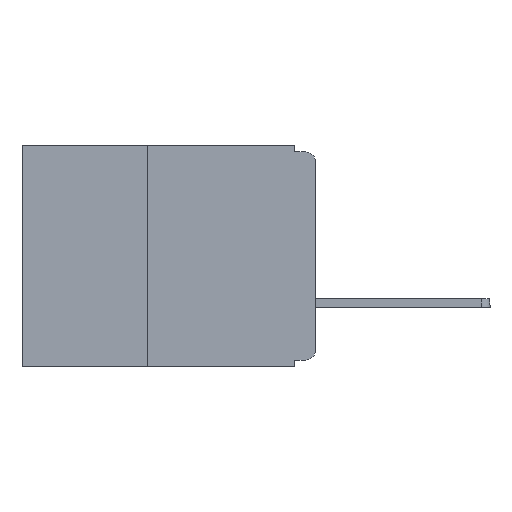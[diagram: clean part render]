
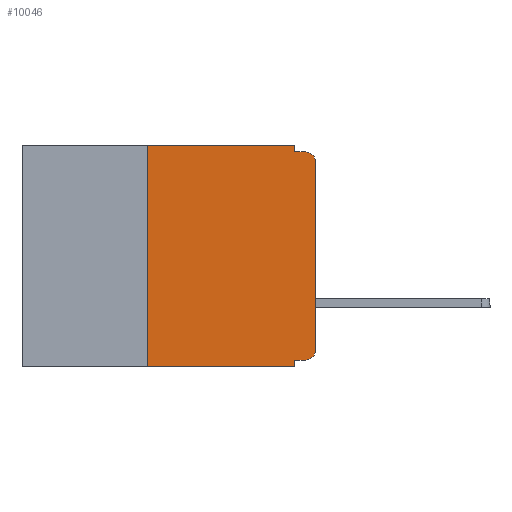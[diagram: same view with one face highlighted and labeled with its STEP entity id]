
A CAD part, left-side view. The second image highlights one B-rep face of the part: STEP entity #10046.
In plain terms, the highlighted planar face has unit normal (-1, 0, 0).
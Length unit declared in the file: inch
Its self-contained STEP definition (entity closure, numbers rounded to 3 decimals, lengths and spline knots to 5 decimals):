
#100 = AXIS2_PLACEMENT_3D ( 'NONE', #8703, #17925, #8762 ) ;
#139 = DIRECTION ( 'NONE',  ( 0., -1., 0. ) ) ;
#202 = EDGE_CURVE ( 'NONE', #17765, #14325, #5514, .T. ) ;
#685 = ORIENTED_EDGE ( 'NONE', *, *, #18045, .T. ) ;
#1117 = DIRECTION ( 'NONE',  ( 0., 0., 1. ) ) ;
#1303 = VERTEX_POINT ( 'NONE', #18175 ) ;
#1497 = LINE ( 'NONE', #11388, #17053 ) ;
#1710 = CARTESIAN_POINT ( 'NONE',  ( 0., 0.031, -0.33 ) ) ;
#2176 = VECTOR ( 'NONE', #14644, 39.37008 ) ;
#2225 = ORIENTED_EDGE ( 'NONE', *, *, #13174, .F. ) ;
#2400 = LINE ( 'NONE', #1710, #6132 ) ;
#2518 = VERTEX_POINT ( 'NONE', #12500 ) ;
#2671 = AXIS2_PLACEMENT_3D ( 'NONE', #9550, #17974, #17884 ) ;
#2777 = EDGE_CURVE ( 'NONE', #10951, #12198, #5656, .T. ) ;
#3231 = CARTESIAN_POINT ( 'NONE',  ( 0., 0., -0.025 ) ) ;
#3248 = ORIENTED_EDGE ( 'NONE', *, *, #9773, .F. ) ;
#3385 = EDGE_CURVE ( 'NONE', #2518, #15820, #14563, .T. ) ;
#3405 = LINE ( 'NONE', #16831, #15208 ) ;
#4497 = DIRECTION ( 'NONE',  ( 0., 1., 0. ) ) ;
#4747 = VERTEX_POINT ( 'NONE', #12526 ) ;
#4952 = ORIENTED_EDGE ( 'NONE', *, *, #2777, .T. ) ;
#5126 = EDGE_CURVE ( 'NONE', #1303, #2518, #15710, .T. ) ;
#5514 = CIRCLE ( 'NONE', #2671, 0.015 ) ;
#5656 = CIRCLE ( 'NONE', #14156, 0.015 ) ;
#5667 = EDGE_LOOP ( 'NONE', ( #685, #4952, #9624, #13665, #18238, #2225, #6457, #3248, #11553, #12018 ) ) ;
#6132 = VECTOR ( 'NONE', #14176, 39.37008 ) ;
#6457 = ORIENTED_EDGE ( 'NONE', *, *, #18872, .T. ) ;
#7185 = PLANE ( 'NONE',  #100 ) ;
#7316 = VERTEX_POINT ( 'NONE', #9727 ) ;
#8703 = CARTESIAN_POINT ( 'NONE',  ( 0., 0.437, 0. ) ) ;
#8762 = DIRECTION ( 'NONE',  ( 0., 0., -1. ) ) ;
#8984 = VECTOR ( 'NONE', #19864, 39.37008 ) ;
#9039 = CARTESIAN_POINT ( 'NONE',  ( 0., 0., 0. ) ) ;
#9550 = CARTESIAN_POINT ( 'NONE',  ( 0., 0.015, -0.305 ) ) ;
#9557 = FACE_OUTER_BOUND ( 'NONE', #5667, .T. ) ;
#9624 = ORIENTED_EDGE ( 'NONE', *, *, #15455, .F. ) ;
#9727 = CARTESIAN_POINT ( 'NONE',  ( 0., 0.25, -0.33 ) ) ;
#9773 = EDGE_CURVE ( 'NONE', #4747, #16534, #2400, .T. ) ;
#9821 = VECTOR ( 'NONE', #13951, 39.37008 ) ;
#10046 = ADVANCED_FACE ( 'NONE', ( #9557 ), #7185, .F. ) ;
#10944 = DIRECTION ( 'NONE',  ( -1., 0., 0. ) ) ;
#10951 = VERTEX_POINT ( 'NONE', #3231 ) ;
#11388 = CARTESIAN_POINT ( 'NONE',  ( 0., 0.437, -0.33 ) ) ;
#11553 = ORIENTED_EDGE ( 'NONE', *, *, #14336, .F. ) ;
#12018 = ORIENTED_EDGE ( 'NONE', *, *, #202, .T. ) ;
#12198 = VERTEX_POINT ( 'NONE', #14188 ) ;
#12500 = CARTESIAN_POINT ( 'NONE',  ( 0., 0.031, 0. ) ) ;
#12526 = CARTESIAN_POINT ( 'NONE',  ( 0., 0.031, -0.32 ) ) ;
#13174 = EDGE_CURVE ( 'NONE', #7316, #1303, #14341, .T. ) ;
#13665 = ORIENTED_EDGE ( 'NONE', *, *, #3385, .F. ) ;
#13672 = CARTESIAN_POINT ( 'NONE',  ( 0., 0., -0.01 ) ) ;
#13676 = VECTOR ( 'NONE', #1117, 39.37008 ) ;
#13951 = DIRECTION ( 'NONE',  ( 0., 0., 1. ) ) ;
#14156 = AXIS2_PLACEMENT_3D ( 'NONE', #18827, #10944, #18949 ) ;
#14157 = LINE ( 'NONE', #9039, #13676 ) ;
#14176 = DIRECTION ( 'NONE',  ( 0., 0., -1. ) ) ;
#14188 = CARTESIAN_POINT ( 'NONE',  ( 0., 0.015, -0.01 ) ) ;
#14325 = VERTEX_POINT ( 'NONE', #19896 ) ;
#14336 = EDGE_CURVE ( 'NONE', #17765, #4747, #3405, .T. ) ;
#14341 = LINE ( 'NONE', #17014, #9821 ) ;
#14563 = LINE ( 'NONE', #16482, #2176 ) ;
#14644 = DIRECTION ( 'NONE',  ( 0., 0., -1. ) ) ;
#14974 = CARTESIAN_POINT ( 'NONE',  ( 0., 0.437, 0. ) ) ;
#15208 = VECTOR ( 'NONE', #4497, 39.37008 ) ;
#15455 = EDGE_CURVE ( 'NONE', #15820, #12198, #17595, .T. ) ;
#15710 = LINE ( 'NONE', #14974, #18864 ) ;
#15820 = VERTEX_POINT ( 'NONE', #16098 ) ;
#15919 = DIRECTION ( 'NONE',  ( 0., -1., 0. ) ) ;
#16098 = CARTESIAN_POINT ( 'NONE',  ( 0., 0.031, -0.01 ) ) ;
#16482 = CARTESIAN_POINT ( 'NONE',  ( 0., 0.031, 0. ) ) ;
#16534 = VERTEX_POINT ( 'NONE', #17926 ) ;
#16831 = CARTESIAN_POINT ( 'NONE',  ( 0., 0., -0.32 ) ) ;
#17014 = CARTESIAN_POINT ( 'NONE',  ( 0., 0.25, -0.33 ) ) ;
#17053 = VECTOR ( 'NONE', #15919, 39.37008 ) ;
#17537 = CARTESIAN_POINT ( 'NONE',  ( 0., 0.015, -0.32 ) ) ;
#17595 = LINE ( 'NONE', #13672, #8984 ) ;
#17765 = VERTEX_POINT ( 'NONE', #17537 ) ;
#17884 = DIRECTION ( 'NONE',  ( 0., 0., -1. ) ) ;
#17925 = DIRECTION ( 'NONE',  ( 1., 0., 0. ) ) ;
#17926 = CARTESIAN_POINT ( 'NONE',  ( 0., 0.031, -0.33 ) ) ;
#17974 = DIRECTION ( 'NONE',  ( -1., 0., 0. ) ) ;
#18045 = EDGE_CURVE ( 'NONE', #14325, #10951, #14157, .T. ) ;
#18175 = CARTESIAN_POINT ( 'NONE',  ( 0., 0.25, 0. ) ) ;
#18238 = ORIENTED_EDGE ( 'NONE', *, *, #5126, .F. ) ;
#18827 = CARTESIAN_POINT ( 'NONE',  ( 0., 0.015, -0.025 ) ) ;
#18864 = VECTOR ( 'NONE', #139, 39.37008 ) ;
#18872 = EDGE_CURVE ( 'NONE', #7316, #16534, #1497, .T. ) ;
#18949 = DIRECTION ( 'NONE',  ( 0., 0., -1. ) ) ;
#19864 = DIRECTION ( 'NONE',  ( 0., -1., 0. ) ) ;
#19896 = CARTESIAN_POINT ( 'NONE',  ( 0., 0., -0.305 ) ) ;
